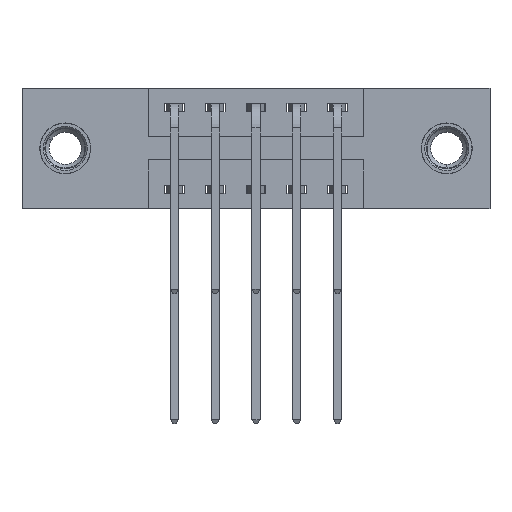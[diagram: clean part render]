
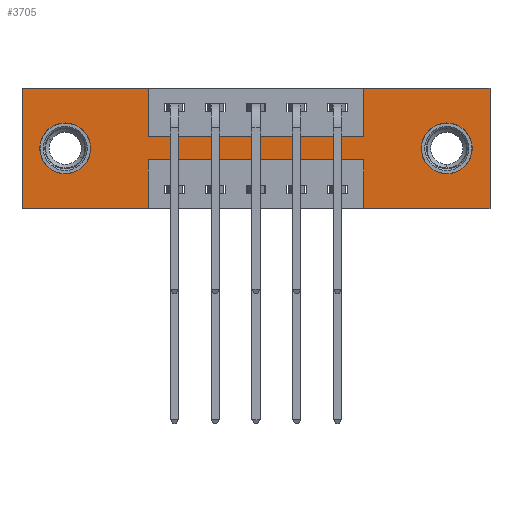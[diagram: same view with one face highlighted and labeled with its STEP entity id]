
A CAD part, front view. The second image highlights one B-rep face of the part: STEP entity #3705.
In plain terms, the highlighted planar face has unit normal (0, -1, 0).
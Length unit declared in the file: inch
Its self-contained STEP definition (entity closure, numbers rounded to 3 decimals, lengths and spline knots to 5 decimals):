
#96 = CARTESIAN_POINT ( 'NONE',  ( 0., 0., 0. ) ) ;
#159 = EDGE_CURVE ( 'NONE', #285, #8061, #6216, .T. ) ;
#241 = EDGE_CURVE ( 'NONE', #10851, #8126, #7553, .T. ) ;
#285 = VERTEX_POINT ( 'NONE', #7448 ) ;
#305 = VERTEX_POINT ( 'NONE', #4778 ) ;
#393 = EDGE_CURVE ( 'NONE', #305, #6111, #5705, .T. ) ;
#411 = LINE ( 'NONE', #10847, #9459 ) ;
#443 = ORIENTED_EDGE ( 'NONE', *, *, #3181, .F. ) ;
#457 = DIRECTION ( 'NONE',  ( 1., 0., 0. ) ) ;
#493 = DIRECTION ( 'NONE',  ( -1., 0., 0. ) ) ;
#627 = DIRECTION ( 'NONE',  ( 0., 0., 1. ) ) ;
#658 = ORIENTED_EDGE ( 'NONE', *, *, #2782, .F. ) ;
#878 = CARTESIAN_POINT ( 'NONE',  ( 1.0475, 0., -0.22 ) ) ;
#899 = VECTOR ( 'NONE', #907, 39.37008 ) ;
#907 = DIRECTION ( 'NONE',  ( 0., 0., -1. ) ) ;
#947 = CARTESIAN_POINT ( 'NONE',  ( 0., 0., 0. ) ) ;
#1333 = DIRECTION ( 'NONE',  ( 0., 0., -1. ) ) ;
#1335 = CARTESIAN_POINT ( 'NONE',  ( 1.3025, 0., -0.263 ) ) ;
#1434 = LINE ( 'NONE', #9183, #8722 ) ;
#1515 = EDGE_LOOP ( 'NONE', ( #10977, #5579 ) ) ;
#1680 = EDGE_CURVE ( 'NONE', #10091, #1830, #9145, .T. ) ;
#1725 = CARTESIAN_POINT ( 'NONE',  ( 0., 0., -0.37 ) ) ;
#1805 = CARTESIAN_POINT ( 'NONE',  ( 0.1325, 0., -0.107 ) ) ;
#1830 = VERTEX_POINT ( 'NONE', #10382 ) ;
#1843 = VERTEX_POINT ( 'NONE', #4234 ) ;
#1866 = CARTESIAN_POINT ( 'NONE',  ( 0.3875, 0., -0.22 ) ) ;
#2033 = ORIENTED_EDGE ( 'NONE', *, *, #393, .T. ) ;
#2123 = CARTESIAN_POINT ( 'NONE',  ( 0., 0., 0. ) ) ;
#2236 = DIRECTION ( 'NONE',  ( 0., 0., 1. ) ) ;
#2248 = DIRECTION ( 'NONE',  ( 0., 0., 1. ) ) ;
#2323 = EDGE_CURVE ( 'NONE', #1843, #5942, #8706, .T. ) ;
#2354 = CIRCLE ( 'NONE', #8528, 0.078 ) ;
#2579 = VERTEX_POINT ( 'NONE', #10753 ) ;
#2596 = ORIENTED_EDGE ( 'NONE', *, *, #4676, .F. ) ;
#2713 = VECTOR ( 'NONE', #2236, 39.37008 ) ;
#2722 = VECTOR ( 'NONE', #7733, 39.37008 ) ;
#2782 = EDGE_CURVE ( 'NONE', #8061, #4532, #4256, .T. ) ;
#2791 = VERTEX_POINT ( 'NONE', #5975 ) ;
#2806 = CARTESIAN_POINT ( 'NONE',  ( 0.3875, 0., 0. ) ) ;
#2876 = AXIS2_PLACEMENT_3D ( 'NONE', #1725, #8569, #10380 ) ;
#3019 = DIRECTION ( 'NONE',  ( 1., 0., 0. ) ) ;
#3025 = LINE ( 'NONE', #8878, #5025 ) ;
#3033 = EDGE_CURVE ( 'NONE', #3348, #10091, #3025, .T. ) ;
#3065 = CARTESIAN_POINT ( 'NONE',  ( 0.3875, 0., -0.37 ) ) ;
#3181 = EDGE_CURVE ( 'NONE', #1830, #285, #5798, .T. ) ;
#3192 = ORIENTED_EDGE ( 'NONE', *, *, #3033, .F. ) ;
#3262 = VECTOR ( 'NONE', #5835, 39.37008 ) ;
#3348 = VERTEX_POINT ( 'NONE', #878 ) ;
#3705 = ADVANCED_FACE ( 'NONE', ( #10483, #5097, #5202 ), #9364, .T. ) ;
#3884 = CARTESIAN_POINT ( 'NONE',  ( 1.0475, 0., -0.37 ) ) ;
#3931 = DIRECTION ( 'NONE',  ( 0., 1., 0. ) ) ;
#4020 = ORIENTED_EDGE ( 'NONE', *, *, #8980, .F. ) ;
#4234 = CARTESIAN_POINT ( 'NONE',  ( 0.1325, 0., -0.263 ) ) ;
#4256 = LINE ( 'NONE', #96, #2722 ) ;
#4338 = AXIS2_PLACEMENT_3D ( 'NONE', #10121, #3931, #9971 ) ;
#4532 = VERTEX_POINT ( 'NONE', #5962 ) ;
#4676 = EDGE_CURVE ( 'NONE', #6951, #6600, #9716, .T. ) ;
#4778 = CARTESIAN_POINT ( 'NONE',  ( 1.3025, 0., -0.107 ) ) ;
#4987 = ORIENTED_EDGE ( 'NONE', *, *, #1680, .F. ) ;
#5025 = VECTOR ( 'NONE', #8086, 39.37008 ) ;
#5097 = FACE_BOUND ( 'NONE', #1515, .T. ) ;
#5202 = FACE_OUTER_BOUND ( 'NONE', #10592, .T. ) ;
#5579 = ORIENTED_EDGE ( 'NONE', *, *, #2323, .T. ) ;
#5705 = CIRCLE ( 'NONE', #11123, 0.078 ) ;
#5798 = LINE ( 'NONE', #7506, #8482 ) ;
#5835 = DIRECTION ( 'NONE',  ( 0., 0., -1. ) ) ;
#5942 = VERTEX_POINT ( 'NONE', #1805 ) ;
#5962 = CARTESIAN_POINT ( 'NONE',  ( 0.3875, 0., 0. ) ) ;
#5975 = CARTESIAN_POINT ( 'NONE',  ( 0.3875, 0., -0.15 ) ) ;
#5984 = CARTESIAN_POINT ( 'NONE',  ( 1.0475, 0., -0.37 ) ) ;
#6016 = DIRECTION ( 'NONE',  ( 0., 0., 1. ) ) ;
#6096 = CARTESIAN_POINT ( 'NONE',  ( 1.0475, 0., 0. ) ) ;
#6111 = VERTEX_POINT ( 'NONE', #1335 ) ;
#6216 = LINE ( 'NONE', #947, #7134 ) ;
#6290 = ORIENTED_EDGE ( 'NONE', *, *, #9309, .F. ) ;
#6526 = AXIS2_PLACEMENT_3D ( 'NONE', #8605, #11202, #627 ) ;
#6600 = VERTEX_POINT ( 'NONE', #9026 ) ;
#6951 = VERTEX_POINT ( 'NONE', #6096 ) ;
#7134 = VECTOR ( 'NONE', #8818, 39.37008 ) ;
#7238 = EDGE_CURVE ( 'NONE', #5942, #1843, #2354, .T. ) ;
#7257 = ORIENTED_EDGE ( 'NONE', *, *, #9174, .F. ) ;
#7375 = LINE ( 'NONE', #10086, #3262 ) ;
#7448 = CARTESIAN_POINT ( 'NONE',  ( 0., 0., -0.37 ) ) ;
#7506 = CARTESIAN_POINT ( 'NONE',  ( 0., 0., -0.37 ) ) ;
#7553 = LINE ( 'NONE', #9108, #8398 ) ;
#7613 = CIRCLE ( 'NONE', #4338, 0.078 ) ;
#7733 = DIRECTION ( 'NONE',  ( 1., 0., 0. ) ) ;
#7842 = DIRECTION ( 'NONE',  ( 0., 0., -1. ) ) ;
#7852 = ORIENTED_EDGE ( 'NONE', *, *, #9039, .F. ) ;
#7939 = EDGE_CURVE ( 'NONE', #6111, #305, #7613, .T. ) ;
#7953 = EDGE_CURVE ( 'NONE', #8126, #3348, #8224, .T. ) ;
#8046 = ORIENTED_EDGE ( 'NONE', *, *, #159, .F. ) ;
#8061 = VERTEX_POINT ( 'NONE', #2123 ) ;
#8086 = DIRECTION ( 'NONE',  ( -1., 0., 0. ) ) ;
#8126 = VERTEX_POINT ( 'NONE', #5984 ) ;
#8224 = LINE ( 'NONE', #3884, #2713 ) ;
#8398 = VECTOR ( 'NONE', #9152, 39.37008 ) ;
#8482 = VECTOR ( 'NONE', #493, 39.37008 ) ;
#8496 = LINE ( 'NONE', #2806, #899 ) ;
#8528 = AXIS2_PLACEMENT_3D ( 'NONE', #9581, #11108, #6016 ) ;
#8536 = VECTOR ( 'NONE', #3019, 39.37008 ) ;
#8569 = DIRECTION ( 'NONE',  ( 0., -1., 0. ) ) ;
#8605 = CARTESIAN_POINT ( 'NONE',  ( 0.1325, 0., -0.185 ) ) ;
#8706 = CIRCLE ( 'NONE', #6526, 0.078 ) ;
#8722 = VECTOR ( 'NONE', #2248, 39.37008 ) ;
#8818 = DIRECTION ( 'NONE',  ( 0., 0., 1. ) ) ;
#8878 = CARTESIAN_POINT ( 'NONE',  ( 0.3875, 0., -0.22 ) ) ;
#8980 = EDGE_CURVE ( 'NONE', #2579, #6951, #1434, .T. ) ;
#9026 = CARTESIAN_POINT ( 'NONE',  ( 1.435, 0., 0. ) ) ;
#9039 = EDGE_CURVE ( 'NONE', #6600, #10851, #7375, .T. ) ;
#9108 = CARTESIAN_POINT ( 'NONE',  ( 0., 0., -0.37 ) ) ;
#9145 = LINE ( 'NONE', #3065, #9782 ) ;
#9152 = DIRECTION ( 'NONE',  ( -1., 0., 0. ) ) ;
#9174 = EDGE_CURVE ( 'NONE', #4532, #2791, #8496, .T. ) ;
#9183 = CARTESIAN_POINT ( 'NONE',  ( 1.0475, 0., 0. ) ) ;
#9309 = EDGE_CURVE ( 'NONE', #2791, #2579, #411, .T. ) ;
#9364 = PLANE ( 'NONE',  #2876 ) ;
#9408 = ORIENTED_EDGE ( 'NONE', *, *, #241, .F. ) ;
#9459 = VECTOR ( 'NONE', #457, 39.37008 ) ;
#9508 = EDGE_LOOP ( 'NONE', ( #2033, #10077 ) ) ;
#9581 = CARTESIAN_POINT ( 'NONE',  ( 0.1325, 0., -0.185 ) ) ;
#9716 = LINE ( 'NONE', #10783, #8536 ) ;
#9782 = VECTOR ( 'NONE', #1333, 39.37008 ) ;
#9971 = DIRECTION ( 'NONE',  ( 0., 0., -1. ) ) ;
#10077 = ORIENTED_EDGE ( 'NONE', *, *, #7939, .T. ) ;
#10086 = CARTESIAN_POINT ( 'NONE',  ( 1.435, 0., 0. ) ) ;
#10091 = VERTEX_POINT ( 'NONE', #1866 ) ;
#10121 = CARTESIAN_POINT ( 'NONE',  ( 1.3025, 0., -0.185 ) ) ;
#10327 = DIRECTION ( 'NONE',  ( 0., 1., 0. ) ) ;
#10380 = DIRECTION ( 'NONE',  ( 0., 0., -1. ) ) ;
#10382 = CARTESIAN_POINT ( 'NONE',  ( 0.3875, 0., -0.37 ) ) ;
#10483 = FACE_BOUND ( 'NONE', #9508, .T. ) ;
#10592 = EDGE_LOOP ( 'NONE', ( #4987, #3192, #10830, #9408, #7852, #2596, #4020, #6290, #7257, #658, #8046, #443 ) ) ;
#10753 = CARTESIAN_POINT ( 'NONE',  ( 1.0475, 0., -0.15 ) ) ;
#10783 = CARTESIAN_POINT ( 'NONE',  ( 0., 0., 0. ) ) ;
#10830 = ORIENTED_EDGE ( 'NONE', *, *, #7953, .F. ) ;
#10847 = CARTESIAN_POINT ( 'NONE',  ( 0.3875, 0., -0.15 ) ) ;
#10851 = VERTEX_POINT ( 'NONE', #10864 ) ;
#10864 = CARTESIAN_POINT ( 'NONE',  ( 1.435, 0., -0.37 ) ) ;
#10977 = ORIENTED_EDGE ( 'NONE', *, *, #7238, .T. ) ;
#11108 = DIRECTION ( 'NONE',  ( 0., 1., 0. ) ) ;
#11123 = AXIS2_PLACEMENT_3D ( 'NONE', #11234, #10327, #7842 ) ;
#11202 = DIRECTION ( 'NONE',  ( 0., 1., 0. ) ) ;
#11234 = CARTESIAN_POINT ( 'NONE',  ( 1.3025, 0., -0.185 ) ) ;
